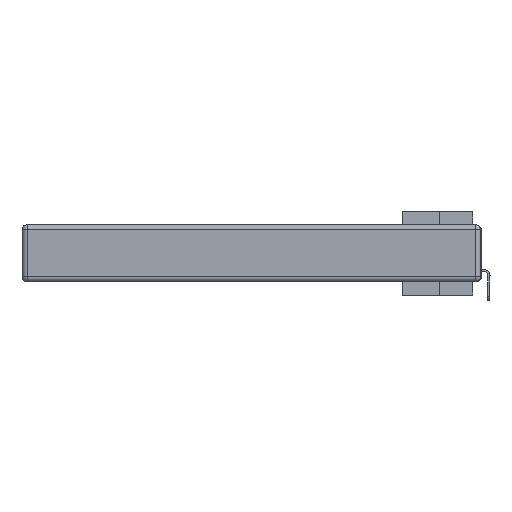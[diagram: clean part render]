
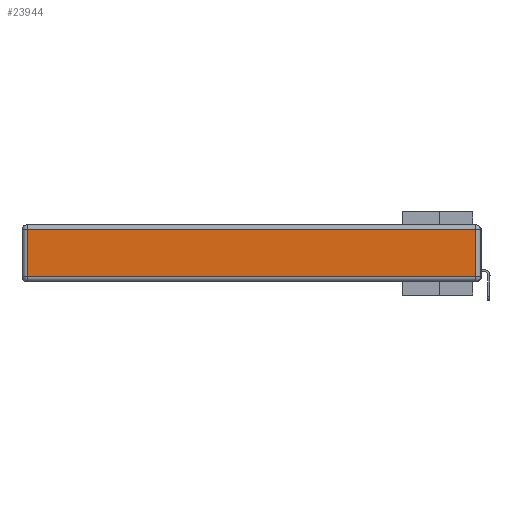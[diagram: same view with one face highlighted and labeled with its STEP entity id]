
A CAD part, left-side view. The second image highlights one B-rep face of the part: STEP entity #23944.
In plain terms, the highlighted planar face has unit normal (-1, 0, 0).
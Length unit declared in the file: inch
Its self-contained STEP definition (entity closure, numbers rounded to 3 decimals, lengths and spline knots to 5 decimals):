
#2891 = CARTESIAN_POINT ( 'NONE',  ( 0., 0., -0.313 ) ) ;
#5694 = CARTESIAN_POINT ( 'NONE',  ( 0., 0.03, -0.343 ) ) ;
#5950 = VERTEX_POINT ( 'NONE', #13415 ) ;
#6240 = VERTEX_POINT ( 'NONE', #27436 ) ;
#6813 = EDGE_CURVE ( 'NONE', #5950, #6240, #22946, .T. ) ;
#8417 = FACE_OUTER_BOUND ( 'NONE', #24784, .T. ) ;
#8622 = CARTESIAN_POINT ( 'NONE',  ( 0., 0., -0.343 ) ) ;
#8651 = VERTEX_POINT ( 'NONE', #38149 ) ;
#13415 = CARTESIAN_POINT ( 'NONE',  ( 0., 2.72, -0.03 ) ) ;
#13601 = EDGE_CURVE ( 'NONE', #6240, #24475, #24171, .T. ) ;
#13879 = ORIENTED_EDGE ( 'NONE', *, *, #33993, .T. ) ;
#18052 = DIRECTION ( 'NONE',  ( 0., 0., 1. ) ) ;
#19354 = VECTOR ( 'NONE', #24370, 39.37008 ) ;
#19432 = VECTOR ( 'NONE', #29750, 39.37008 ) ;
#19445 = DIRECTION ( 'NONE',  ( 0., 1., 0. ) ) ;
#22020 = ORIENTED_EDGE ( 'NONE', *, *, #13601, .T. ) ;
#22152 = DIRECTION ( 'NONE',  ( 0., 0., -1. ) ) ;
#22545 = CARTESIAN_POINT ( 'NONE',  ( 0., 2.72, -0.343 ) ) ;
#22575 = ORIENTED_EDGE ( 'NONE', *, *, #6813, .T. ) ;
#22946 = LINE ( 'NONE', #22545, #24983 ) ;
#23944 = ADVANCED_FACE ( 'NONE', ( #8417 ), #26487, .T. ) ;
#24171 = LINE ( 'NONE', #2891, #19354 ) ;
#24370 = DIRECTION ( 'NONE',  ( 0., -1., 0. ) ) ;
#24475 = VERTEX_POINT ( 'NONE', #27765 ) ;
#24784 = EDGE_LOOP ( 'NONE', ( #22020, #29230, #13879, #22575 ) ) ;
#24983 = VECTOR ( 'NONE', #22152, 39.37008 ) ;
#26487 = PLANE ( 'NONE',  #37824 ) ;
#27436 = CARTESIAN_POINT ( 'NONE',  ( 0., 2.72, -0.313 ) ) ;
#27765 = CARTESIAN_POINT ( 'NONE',  ( 0., 0.03, -0.313 ) ) ;
#29230 = ORIENTED_EDGE ( 'NONE', *, *, #38743, .T. ) ;
#29679 = DIRECTION ( 'NONE',  ( -1., 0., 0. ) ) ;
#29750 = DIRECTION ( 'NONE',  ( 0., 0., 1. ) ) ;
#31656 = CARTESIAN_POINT ( 'NONE',  ( 0., 2.75, -0.03 ) ) ;
#32246 = LINE ( 'NONE', #31656, #36682 ) ;
#33139 = LINE ( 'NONE', #5694, #19432 ) ;
#33993 = EDGE_CURVE ( 'NONE', #8651, #5950, #32246, .T. ) ;
#36682 = VECTOR ( 'NONE', #19445, 39.37008 ) ;
#37824 = AXIS2_PLACEMENT_3D ( 'NONE', #8622, #29679, #18052 ) ;
#38149 = CARTESIAN_POINT ( 'NONE',  ( 0., 0.03, -0.03 ) ) ;
#38743 = EDGE_CURVE ( 'NONE', #24475, #8651, #33139, .T. ) ;
